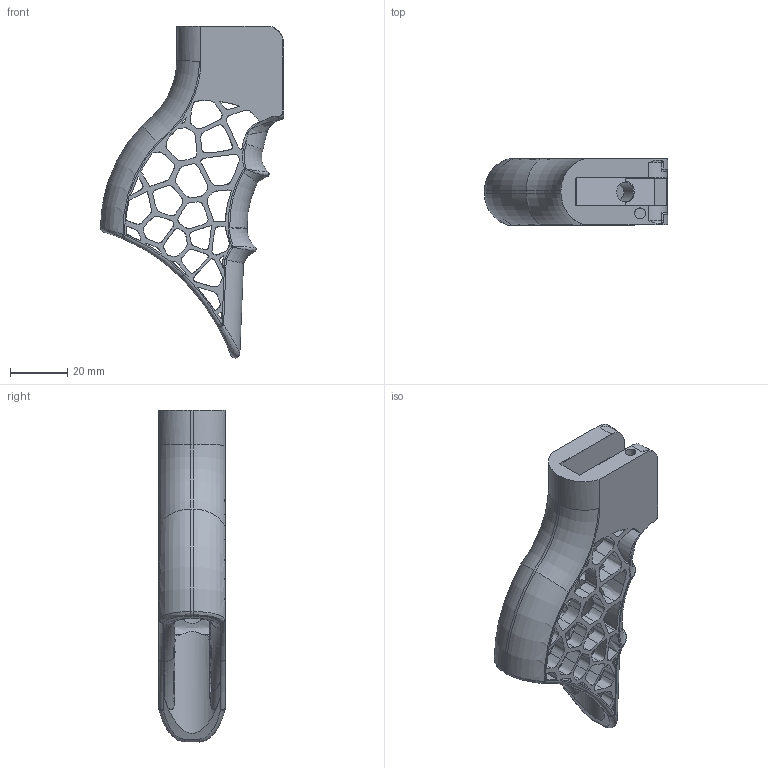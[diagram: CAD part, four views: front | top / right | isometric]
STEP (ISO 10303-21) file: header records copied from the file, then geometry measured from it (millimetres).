
FILE_DESCRIPTION(/* description */ (''),/* implementation_level */ '2;1');
FILE_NAME(/* name */ 'grip.step',/* time_stamp */ '2021-09-02T19:33:08-05:00',/* author */ (''),/* organization */ (''),/* preprocessor_version */ 'ST-DEVELOPER v18.1',/* originating_system */ 'Autodesk Translation Framework v10.10.0.1391',/* authorisation */ '');
FILE_SCHEMA (('AUTOMOTIVE_DESIGN { 1 0 10303 214 3 1 1 }'));
Products named in the file (1): grip
Bounding box: 63.75 x 23.02 x 115.51 mm (x, y, z)
Volume: 42314.6 mm3; surface area: 22410.7 mm2
Topology: 1 solids, 1 shells, 447 faces, 1411 edges, 927 vertices
Faces by surface type: bspline 288, cylinder 66, plane 47, torus 40, sphere 5, cone 1
Full cylindrical faces by diameter (mm): 3.75 x1, 6.8 x1
Entity records: 40128 total; most frequent: CARTESIAN_POINT 29683, ORIENTED_EDGE 2818, EDGE_CURVE 1409, DIRECTION 1128, VERTEX_POINT 927, B_SPLINE_CURVE_WITH_KNOTS 776, EDGE_LOOP 516, LINE 450
